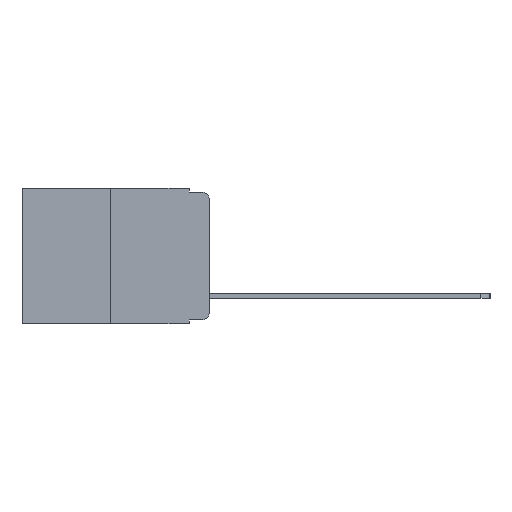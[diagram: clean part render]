
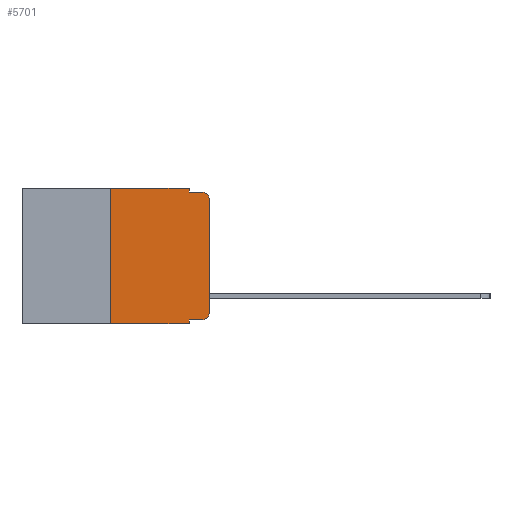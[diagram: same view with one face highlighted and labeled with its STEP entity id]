
A CAD part, left-side view. The second image highlights one B-rep face of the part: STEP entity #5701.
In plain terms, the highlighted planar face has unit normal (-1, 0, 0).
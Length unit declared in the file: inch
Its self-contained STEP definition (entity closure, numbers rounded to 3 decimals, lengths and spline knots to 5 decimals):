
#33 = VERTEX_POINT ( 'NONE', #11174 ) ;
#273 = ORIENTED_EDGE ( 'NONE', *, *, #4235, .T. ) ;
#301 = DIRECTION ( 'NONE',  ( -1., 0., 0. ) ) ;
#720 = EDGE_CURVE ( 'NONE', #8392, #2826, #4608, .T. ) ;
#856 = ORIENTED_EDGE ( 'NONE', *, *, #9336, .F. ) ;
#988 = CARTESIAN_POINT ( 'NONE',  ( 0., 0., -0.313 ) ) ;
#1015 = ORIENTED_EDGE ( 'NONE', *, *, #10885, .F. ) ;
#1439 = CARTESIAN_POINT ( 'NONE',  ( 0., 0.25, 0. ) ) ;
#1472 = CARTESIAN_POINT ( 'NONE',  ( 0., 0.051, -0.01 ) ) ;
#1644 = CARTESIAN_POINT ( 'NONE',  ( 0., 0.25, 0. ) ) ;
#1757 = CARTESIAN_POINT ( 'NONE',  ( 0., 0.473, -0.343 ) ) ;
#1882 = EDGE_CURVE ( 'NONE', #2826, #33, #3202, .T. ) ;
#1918 = ORIENTED_EDGE ( 'NONE', *, *, #4487, .T. ) ;
#2539 = CARTESIAN_POINT ( 'NONE',  ( 0., 0.25, -0.343 ) ) ;
#2600 = LINE ( 'NONE', #6383, #9215 ) ;
#2651 = ORIENTED_EDGE ( 'NONE', *, *, #720, .F. ) ;
#2732 = VECTOR ( 'NONE', #5900, 39.37008 ) ;
#2779 = DIRECTION ( 'NONE',  ( 0., 0., -1. ) ) ;
#2795 = VECTOR ( 'NONE', #2779, 39.37008 ) ;
#2826 = VERTEX_POINT ( 'NONE', #1644 ) ;
#2933 = VECTOR ( 'NONE', #7470, 39.37008 ) ;
#2993 = DIRECTION ( 'NONE',  ( 1., 0., 0. ) ) ;
#3074 = CARTESIAN_POINT ( 'NONE',  ( 0., 0., 0. ) ) ;
#3202 = LINE ( 'NONE', #4911, #2933 ) ;
#3566 = ORIENTED_EDGE ( 'NONE', *, *, #7507, .T. ) ;
#3823 = CARTESIAN_POINT ( 'NONE',  ( 0., 0.02, -0.03 ) ) ;
#3885 = LINE ( 'NONE', #3074, #8480 ) ;
#3973 = DIRECTION ( 'NONE',  ( 0., 0., -1. ) ) ;
#4143 = CIRCLE ( 'NONE', #10270, 0.02 ) ;
#4183 = EDGE_CURVE ( 'NONE', #4850, #6760, #9405, .T. ) ;
#4235 = EDGE_CURVE ( 'NONE', #11024, #4693, #8631, .T. ) ;
#4436 = EDGE_LOOP ( 'NONE', ( #1918, #273, #856, #1015, #7081, #2651, #9534, #8755, #9890, #3566 ) ) ;
#4459 = VERTEX_POINT ( 'NONE', #5709 ) ;
#4487 = EDGE_CURVE ( 'NONE', #4812, #11024, #3885, .T. ) ;
#4608 = LINE ( 'NONE', #1439, #6615 ) ;
#4613 = CARTESIAN_POINT ( 'NONE',  ( 0., 0.473, 0. ) ) ;
#4693 = VERTEX_POINT ( 'NONE', #8655 ) ;
#4714 = VERTEX_POINT ( 'NONE', #1472 ) ;
#4772 = EDGE_CURVE ( 'NONE', #8392, #6760, #9790, .T. ) ;
#4812 = VERTEX_POINT ( 'NONE', #988 ) ;
#4850 = VERTEX_POINT ( 'NONE', #5422 ) ;
#4911 = CARTESIAN_POINT ( 'NONE',  ( 0., 0.473, 0. ) ) ;
#4912 = PLANE ( 'NONE',  #8158 ) ;
#5422 = CARTESIAN_POINT ( 'NONE',  ( 0., 0.051, -0.333 ) ) ;
#5583 = DIRECTION ( 'NONE',  ( 0., 0., 1. ) ) ;
#5650 = CARTESIAN_POINT ( 'NONE',  ( 0., 0.02, -0.313 ) ) ;
#5701 = ADVANCED_FACE ( 'NONE', ( #7240 ), #4912, .F. ) ;
#5709 = CARTESIAN_POINT ( 'NONE',  ( 0., 0.02, -0.333 ) ) ;
#5900 = DIRECTION ( 'NONE',  ( 0., -1., 0. ) ) ;
#6294 = CARTESIAN_POINT ( 'NONE',  ( 0., 0.051, 0. ) ) ;
#6383 = CARTESIAN_POINT ( 'NONE',  ( 0., 0.051, -0.01 ) ) ;
#6456 = CARTESIAN_POINT ( 'NONE',  ( 0., 0.051, 0. ) ) ;
#6501 = DIRECTION ( 'NONE',  ( 0., 0., -1. ) ) ;
#6520 = CARTESIAN_POINT ( 'NONE',  ( 0., 0., -0.03 ) ) ;
#6615 = VECTOR ( 'NONE', #8672, 39.37008 ) ;
#6760 = VERTEX_POINT ( 'NONE', #10214 ) ;
#7081 = ORIENTED_EDGE ( 'NONE', *, *, #1882, .F. ) ;
#7240 = FACE_OUTER_BOUND ( 'NONE', #4436, .T. ) ;
#7267 = VECTOR ( 'NONE', #10025, 39.37008 ) ;
#7356 = LINE ( 'NONE', #10112, #2732 ) ;
#7470 = DIRECTION ( 'NONE',  ( 0., -1., 0. ) ) ;
#7507 = EDGE_CURVE ( 'NONE', #4459, #4812, #4143, .T. ) ;
#8075 = AXIS2_PLACEMENT_3D ( 'NONE', #3823, #9004, #9911 ) ;
#8158 = AXIS2_PLACEMENT_3D ( 'NONE', #4613, #2993, #3973 ) ;
#8392 = VERTEX_POINT ( 'NONE', #2539 ) ;
#8480 = VECTOR ( 'NONE', #5583, 39.37008 ) ;
#8631 = CIRCLE ( 'NONE', #8075, 0.02 ) ;
#8655 = CARTESIAN_POINT ( 'NONE',  ( 0., 0.02, -0.01 ) ) ;
#8672 = DIRECTION ( 'NONE',  ( 0., 0., 1. ) ) ;
#8755 = ORIENTED_EDGE ( 'NONE', *, *, #4183, .F. ) ;
#9004 = DIRECTION ( 'NONE',  ( -1., 0., 0. ) ) ;
#9065 = VECTOR ( 'NONE', #10577, 39.37008 ) ;
#9215 = VECTOR ( 'NONE', #9835, 39.37008 ) ;
#9336 = EDGE_CURVE ( 'NONE', #4714, #4693, #2600, .T. ) ;
#9405 = LINE ( 'NONE', #6456, #2795 ) ;
#9534 = ORIENTED_EDGE ( 'NONE', *, *, #4772, .T. ) ;
#9790 = LINE ( 'NONE', #1757, #7267 ) ;
#9821 = LINE ( 'NONE', #6294, #9065 ) ;
#9835 = DIRECTION ( 'NONE',  ( 0., -1., 0. ) ) ;
#9890 = ORIENTED_EDGE ( 'NONE', *, *, #9926, .T. ) ;
#9911 = DIRECTION ( 'NONE',  ( 0., 0., -1. ) ) ;
#9926 = EDGE_CURVE ( 'NONE', #4850, #4459, #7356, .T. ) ;
#10025 = DIRECTION ( 'NONE',  ( 0., -1., 0. ) ) ;
#10112 = CARTESIAN_POINT ( 'NONE',  ( 0., 0.051, -0.333 ) ) ;
#10214 = CARTESIAN_POINT ( 'NONE',  ( 0., 0.051, -0.343 ) ) ;
#10270 = AXIS2_PLACEMENT_3D ( 'NONE', #5650, #301, #6501 ) ;
#10577 = DIRECTION ( 'NONE',  ( 0., 0., -1. ) ) ;
#10885 = EDGE_CURVE ( 'NONE', #33, #4714, #9821, .T. ) ;
#11024 = VERTEX_POINT ( 'NONE', #6520 ) ;
#11174 = CARTESIAN_POINT ( 'NONE',  ( 0., 0.051, 0. ) ) ;
